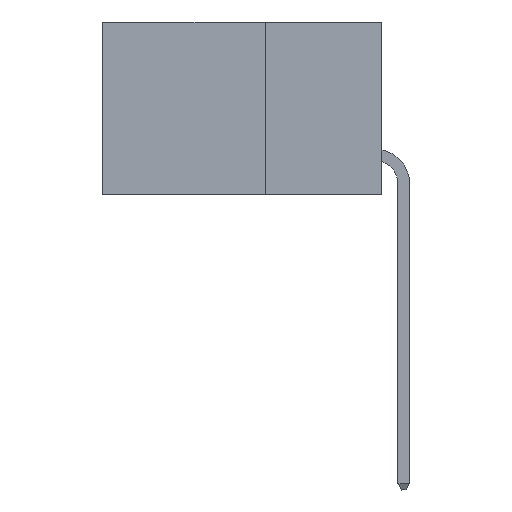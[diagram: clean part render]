
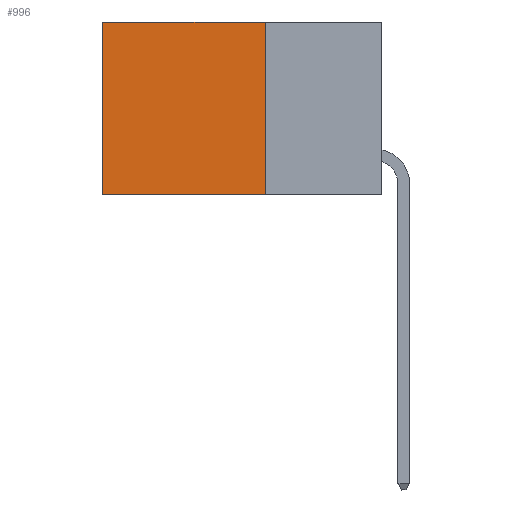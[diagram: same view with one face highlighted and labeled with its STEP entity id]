
A CAD part, left-side view. The second image highlights one B-rep face of the part: STEP entity #996.
In plain terms, the highlighted planar face has unit normal (-1, 0, 0).
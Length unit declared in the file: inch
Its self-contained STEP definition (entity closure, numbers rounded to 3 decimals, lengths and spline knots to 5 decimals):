
#818 = VERTEX_POINT ( 'NONE', #13745 ) ;
#996 = ADVANCED_FACE ( 'NONE', ( #9128 ), #10544, .F. ) ;
#1079 = VECTOR ( 'NONE', #15049, 39.37008 ) ;
#2239 = CARTESIAN_POINT ( 'NONE',  ( 0.2875, 0.25, 0. ) ) ;
#3042 = ORIENTED_EDGE ( 'NONE', *, *, #3737, .F. ) ;
#3314 = ORIENTED_EDGE ( 'NONE', *, *, #19426, .T. ) ;
#3737 = EDGE_CURVE ( 'NONE', #7964, #23019, #4404, .T. ) ;
#4404 = LINE ( 'NONE', #14159, #6965 ) ;
#4762 = EDGE_LOOP ( 'NONE', ( #23505, #3042, #7800, #3314 ) ) ;
#4912 = DIRECTION ( 'NONE',  ( 1., 0., 0. ) ) ;
#5133 = VECTOR ( 'NONE', #20872, 39.37008 ) ;
#6093 = CARTESIAN_POINT ( 'NONE',  ( 0.2875, 0.25, -0.37 ) ) ;
#6821 = CARTESIAN_POINT ( 'NONE',  ( 0.2875, 0.25, 0. ) ) ;
#6965 = VECTOR ( 'NONE', #13836, 39.37008 ) ;
#7800 = ORIENTED_EDGE ( 'NONE', *, *, #22881, .F. ) ;
#7964 = VERTEX_POINT ( 'NONE', #6093 ) ;
#8541 = CARTESIAN_POINT ( 'NONE',  ( 0.2875, 0.6, -0.37 ) ) ;
#9128 = FACE_OUTER_BOUND ( 'NONE', #4762, .T. ) ;
#10492 = CARTESIAN_POINT ( 'NONE',  ( 0.2875, 0.6, 0. ) ) ;
#10522 = AXIS2_PLACEMENT_3D ( 'NONE', #6821, #4912, #17849 ) ;
#10544 = PLANE ( 'NONE',  #10522 ) ;
#12057 = LINE ( 'NONE', #22627, #5133 ) ;
#13014 = VECTOR ( 'NONE', #22579, 39.37008 ) ;
#13745 = CARTESIAN_POINT ( 'NONE',  ( 0.2875, 0.25, 0. ) ) ;
#13836 = DIRECTION ( 'NONE',  ( 0., 1., 0. ) ) ;
#14159 = CARTESIAN_POINT ( 'NONE',  ( 0.2875, 0.25, -0.37 ) ) ;
#15049 = DIRECTION ( 'NONE',  ( 0., 1., 0. ) ) ;
#15462 = CARTESIAN_POINT ( 'NONE',  ( 0.2875, 0.6, 0. ) ) ;
#15657 = LINE ( 'NONE', #2239, #1079 ) ;
#17811 = LINE ( 'NONE', #15462, #13014 ) ;
#17849 = DIRECTION ( 'NONE',  ( 0., 0., -1. ) ) ;
#18857 = EDGE_CURVE ( 'NONE', #21935, #23019, #17811, .T. ) ;
#19426 = EDGE_CURVE ( 'NONE', #818, #21935, #15657, .T. ) ;
#20872 = DIRECTION ( 'NONE',  ( 0., 0., -1. ) ) ;
#21935 = VERTEX_POINT ( 'NONE', #10492 ) ;
#22579 = DIRECTION ( 'NONE',  ( 0., 0., -1. ) ) ;
#22627 = CARTESIAN_POINT ( 'NONE',  ( 0.2875, 0.25, 0. ) ) ;
#22881 = EDGE_CURVE ( 'NONE', #818, #7964, #12057, .T. ) ;
#23019 = VERTEX_POINT ( 'NONE', #8541 ) ;
#23505 = ORIENTED_EDGE ( 'NONE', *, *, #18857, .T. ) ;
